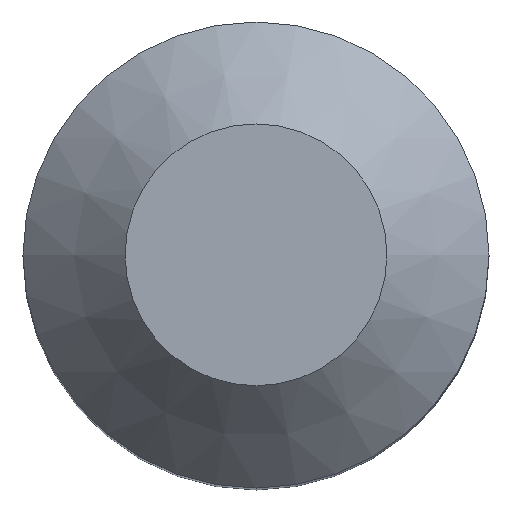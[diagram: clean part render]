
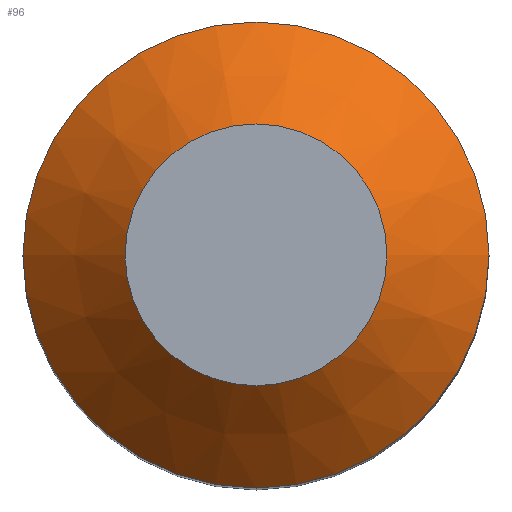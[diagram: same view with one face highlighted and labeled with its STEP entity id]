
A CAD part, top view. The second image highlights one B-rep face of the part: STEP entity #96.
In plain terms, the highlighted conical face has half-angle 45 degrees and reference radius 4.254 mm.
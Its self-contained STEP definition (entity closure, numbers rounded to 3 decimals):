
#16=CONICAL_SURFACE('',#123,4.254,0.785);
#19=LINE('',#208,#22);
#22=VECTOR('',#153,4.254);
#32=FACE_OUTER_BOUND('',#39,.T.);
#39=EDGE_LOOP('',(#84,#85,#86,#87));
#49=CIRCLE('',#122,3.75);
#50=CIRCLE('',#124,2.107);
#56=VERTEX_POINT('',#203);
#57=VERTEX_POINT('',#207);
#66=EDGE_CURVE('',#56,#56,#49,.T.);
#67=EDGE_CURVE('',#56,#57,#19,.T.);
#68=EDGE_CURVE('',#57,#57,#50,.F.);
#84=ORIENTED_EDGE('',*,*,#66,.F.);
#85=ORIENTED_EDGE('',*,*,#67,.T.);
#86=ORIENTED_EDGE('',*,*,#68,.T.);
#87=ORIENTED_EDGE('',*,*,#67,.F.);
#96=ADVANCED_FACE('',(#32),#16,.T.);
#122=AXIS2_PLACEMENT_3D('',#205,#149,#150);
#123=AXIS2_PLACEMENT_3D('',#206,#151,#152);
#124=AXIS2_PLACEMENT_3D('',#209,#154,#155);
#149=DIRECTION('center_axis',(0.,0.,
-1.));
#150=DIRECTION('ref_axis',(-1.,0.,0.));
#151=DIRECTION('center_axis',(0.,0.,
-1.));
#152=DIRECTION('ref_axis',(-1.,0.,0.));
#153=DIRECTION('',(-0.707,0.,0.707));
#154=DIRECTION('center_axis',(0.,0.,
1.));
#155=DIRECTION('ref_axis',(-1.,0.,0.));
#203=CARTESIAN_POINT('',(24.25,0.,-2.643));
#205=CARTESIAN_POINT('Origin',(20.5,0.,-2.643));
#206=CARTESIAN_POINT('Origin',(20.5,0.,-3.146));
#207=CARTESIAN_POINT('',(22.607,0.,-1.));
#208=CARTESIAN_POINT('',(24.754,0.,-3.146));
#209=CARTESIAN_POINT('Origin',(20.5,0.,-1.));
